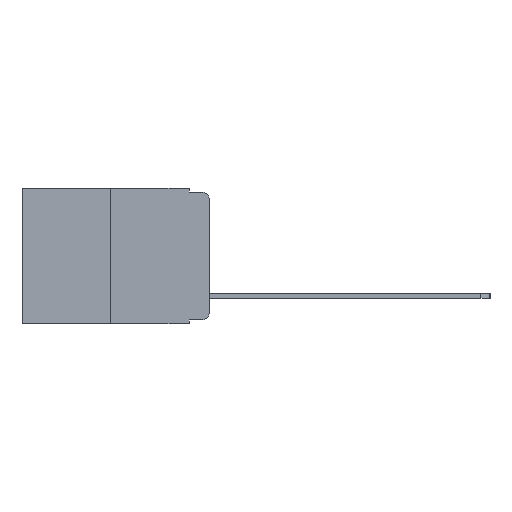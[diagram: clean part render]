
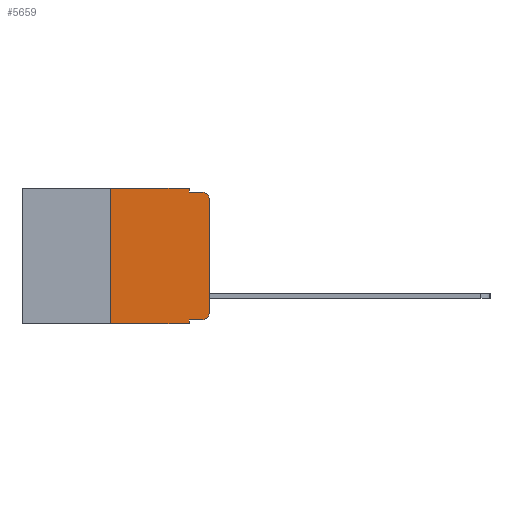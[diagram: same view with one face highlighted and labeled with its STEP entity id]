
A CAD part, left-side view. The second image highlights one B-rep face of the part: STEP entity #5659.
In plain terms, the highlighted planar face has unit normal (-1, 0, 0).
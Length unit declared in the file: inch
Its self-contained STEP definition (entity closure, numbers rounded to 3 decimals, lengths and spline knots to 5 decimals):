
#277 = VECTOR ( 'NONE', #3294, 39.37008 ) ;
#296 = EDGE_LOOP ( 'NONE', ( #11970, #17491, #4485, #7203, #1241, #16296, #10982, #4502, #13453, #10179 ) ) ;
#369 = CARTESIAN_POINT ( 'NONE',  ( 0., 0.02, -0.03 ) ) ;
#524 = EDGE_CURVE ( 'NONE', #12165, #5261, #9371, .T. ) ;
#1000 = CARTESIAN_POINT ( 'NONE',  ( 0., 0.051, -0.01 ) ) ;
#1001 = FACE_OUTER_BOUND ( 'NONE', #296, .T. ) ;
#1073 = EDGE_CURVE ( 'NONE', #5261, #4841, #5433, .T. ) ;
#1241 = ORIENTED_EDGE ( 'NONE', *, *, #1073, .F. ) ;
#1256 = VERTEX_POINT ( 'NONE', #1000 ) ;
#1597 = EDGE_CURVE ( 'NONE', #4841, #1256, #15685, .T. ) ;
#1806 = CARTESIAN_POINT ( 'NONE',  ( 0., 0., 0. ) ) ;
#1987 = DIRECTION ( 'NONE',  ( 0., 0., -1. ) ) ;
#2627 = EDGE_CURVE ( 'NONE', #1256, #14639, #8040, .T. ) ;
#2809 = LINE ( 'NONE', #11641, #16416 ) ;
#3086 = DIRECTION ( 'NONE',  ( 0., -1., 0. ) ) ;
#3294 = DIRECTION ( 'NONE',  ( 0., 0., 1. ) ) ;
#3595 = EDGE_CURVE ( 'NONE', #15408, #14639, #11100, .T. ) ;
#3781 = AXIS2_PLACEMENT_3D ( 'NONE', #369, #10420, #1987 ) ;
#3798 = VERTEX_POINT ( 'NONE', #11050 ) ;
#4117 = PLANE ( 'NONE',  #4666 ) ;
#4236 = CARTESIAN_POINT ( 'NONE',  ( 0., 0., -0.313 ) ) ;
#4304 = LINE ( 'NONE', #1806, #277 ) ;
#4327 = CARTESIAN_POINT ( 'NONE',  ( 0., 0.02, -0.01 ) ) ;
#4485 = ORIENTED_EDGE ( 'NONE', *, *, #2627, .F. ) ;
#4502 = ORIENTED_EDGE ( 'NONE', *, *, #16609, .F. ) ;
#4562 = EDGE_CURVE ( 'NONE', #7251, #15408, #4304, .T. ) ;
#4666 = AXIS2_PLACEMENT_3D ( 'NONE', #13669, #5582, #14975 ) ;
#4711 = VECTOR ( 'NONE', #10413, 39.37008 ) ;
#4841 = VERTEX_POINT ( 'NONE', #5873 ) ;
#5261 = VERTEX_POINT ( 'NONE', #15053 ) ;
#5398 = CARTESIAN_POINT ( 'NONE',  ( 0., 0.02, -0.313 ) ) ;
#5433 = LINE ( 'NONE', #14257, #13040 ) ;
#5582 = DIRECTION ( 'NONE',  ( 1., 0., 0. ) ) ;
#5659 = ADVANCED_FACE ( 'NONE', ( #1001 ), #4117, .F. ) ;
#5778 = CARTESIAN_POINT ( 'NONE',  ( 0., 0., -0.03 ) ) ;
#5873 = CARTESIAN_POINT ( 'NONE',  ( 0., 0.051, 0. ) ) ;
#5945 = CARTESIAN_POINT ( 'NONE',  ( 0., 0.051, -0.01 ) ) ;
#6012 = DIRECTION ( 'NONE',  ( 0., 0., 1. ) ) ;
#6713 = VECTOR ( 'NONE', #3086, 39.37008 ) ;
#6853 = DIRECTION ( 'NONE',  ( 0., 0., -1. ) ) ;
#7062 = DIRECTION ( 'NONE',  ( 0., -1., 0. ) ) ;
#7203 = ORIENTED_EDGE ( 'NONE', *, *, #1597, .F. ) ;
#7251 = VERTEX_POINT ( 'NONE', #4236 ) ;
#8040 = LINE ( 'NONE', #5945, #6713 ) ;
#8239 = VERTEX_POINT ( 'NONE', #15511 ) ;
#8971 = VECTOR ( 'NONE', #6012, 39.37008 ) ;
#9055 = LINE ( 'NONE', #12069, #12120 ) ;
#9371 = LINE ( 'NONE', #14811, #8971 ) ;
#9596 = CARTESIAN_POINT ( 'NONE',  ( 0., 0.02, -0.333 ) ) ;
#10179 = ORIENTED_EDGE ( 'NONE', *, *, #13107, .T. ) ;
#10413 = DIRECTION ( 'NONE',  ( 0., -1., 0. ) ) ;
#10420 = DIRECTION ( 'NONE',  ( -1., 0., 0. ) ) ;
#10982 = ORIENTED_EDGE ( 'NONE', *, *, #17715, .T. ) ;
#11050 = CARTESIAN_POINT ( 'NONE',  ( 0., 0.051, -0.333 ) ) ;
#11100 = CIRCLE ( 'NONE', #3781, 0.02 ) ;
#11146 = CIRCLE ( 'NONE', #17738, 0.02 ) ;
#11641 = CARTESIAN_POINT ( 'NONE',  ( 0., 0.473, -0.343 ) ) ;
#11970 = ORIENTED_EDGE ( 'NONE', *, *, #4562, .T. ) ;
#12069 = CARTESIAN_POINT ( 'NONE',  ( 0., 0.051, 0. ) ) ;
#12120 = VECTOR ( 'NONE', #13410, 39.37008 ) ;
#12165 = VERTEX_POINT ( 'NONE', #17902 ) ;
#12183 = VECTOR ( 'NONE', #12340, 39.37008 ) ;
#12340 = DIRECTION ( 'NONE',  ( 0., 0., -1. ) ) ;
#12389 = LINE ( 'NONE', #12974, #4711 ) ;
#12974 = CARTESIAN_POINT ( 'NONE',  ( 0., 0.051, -0.333 ) ) ;
#13040 = VECTOR ( 'NONE', #7062, 39.37008 ) ;
#13107 = EDGE_CURVE ( 'NONE', #14486, #7251, #11146, .T. ) ;
#13410 = DIRECTION ( 'NONE',  ( 0., 0., -1. ) ) ;
#13453 = ORIENTED_EDGE ( 'NONE', *, *, #14877, .T. ) ;
#13669 = CARTESIAN_POINT ( 'NONE',  ( 0., 0.473, 0. ) ) ;
#14257 = CARTESIAN_POINT ( 'NONE',  ( 0., 0.473, 0. ) ) ;
#14486 = VERTEX_POINT ( 'NONE', #9596 ) ;
#14639 = VERTEX_POINT ( 'NONE', #4327 ) ;
#14806 = DIRECTION ( 'NONE',  ( -1., 0., 0. ) ) ;
#14811 = CARTESIAN_POINT ( 'NONE',  ( 0., 0.25, 0. ) ) ;
#14877 = EDGE_CURVE ( 'NONE', #3798, #14486, #12389, .T. ) ;
#14975 = DIRECTION ( 'NONE',  ( 0., 0., -1. ) ) ;
#15053 = CARTESIAN_POINT ( 'NONE',  ( 0., 0.25, 0. ) ) ;
#15408 = VERTEX_POINT ( 'NONE', #5778 ) ;
#15511 = CARTESIAN_POINT ( 'NONE',  ( 0., 0.051, -0.343 ) ) ;
#15685 = LINE ( 'NONE', #16581, #12183 ) ;
#16296 = ORIENTED_EDGE ( 'NONE', *, *, #524, .F. ) ;
#16416 = VECTOR ( 'NONE', #16837, 39.37008 ) ;
#16581 = CARTESIAN_POINT ( 'NONE',  ( 0., 0.051, 0. ) ) ;
#16609 = EDGE_CURVE ( 'NONE', #3798, #8239, #9055, .T. ) ;
#16837 = DIRECTION ( 'NONE',  ( 0., -1., 0. ) ) ;
#17491 = ORIENTED_EDGE ( 'NONE', *, *, #3595, .T. ) ;
#17715 = EDGE_CURVE ( 'NONE', #12165, #8239, #2809, .T. ) ;
#17738 = AXIS2_PLACEMENT_3D ( 'NONE', #5398, #14806, #6853 ) ;
#17902 = CARTESIAN_POINT ( 'NONE',  ( 0., 0.25, -0.343 ) ) ;
